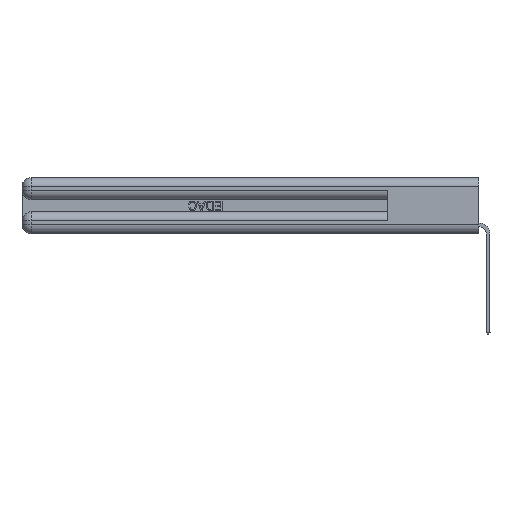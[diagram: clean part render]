
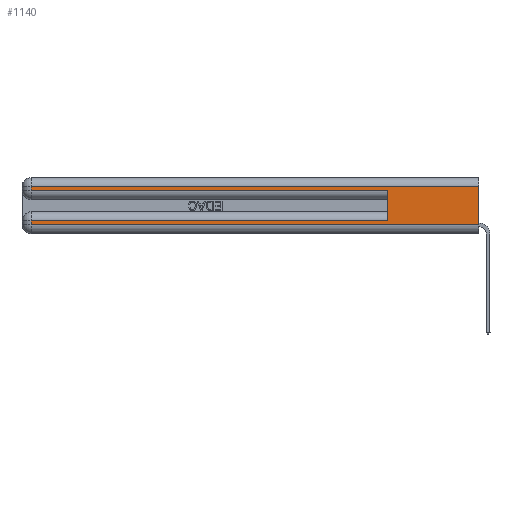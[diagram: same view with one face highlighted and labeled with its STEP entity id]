
A CAD part, left-side view. The second image highlights one B-rep face of the part: STEP entity #1140.
In plain terms, the highlighted planar face has unit normal (-1, 0, 0).
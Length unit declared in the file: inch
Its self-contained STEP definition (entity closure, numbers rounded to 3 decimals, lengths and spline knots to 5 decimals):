
#149 = VERTEX_POINT ( 'NONE', #10172 ) ;
#1140 = ADVANCED_FACE ( 'NONE', ( #12728 ), #4975, .F. ) ;
#1617 = VERTEX_POINT ( 'NONE', #30118 ) ;
#2623 = CARTESIAN_POINT ( 'NONE',  ( 0., 0., 0.06 ) ) ;
#4457 = LINE ( 'NONE', #31286, #9671 ) ;
#4912 = VERTEX_POINT ( 'NONE', #27541 ) ;
#4975 = PLANE ( 'NONE',  #32901 ) ;
#6109 = VECTOR ( 'NONE', #21089, 39.37008 ) ;
#6160 = ORIENTED_EDGE ( 'NONE', *, *, #14109, .T. ) ;
#6341 = ORIENTED_EDGE ( 'NONE', *, *, #18902, .T. ) ;
#6410 = VERTEX_POINT ( 'NONE', #9986 ) ;
#7077 = EDGE_CURVE ( 'NONE', #149, #32841, #21842, .T. ) ;
#7420 = DIRECTION ( 'NONE',  ( 0., -1., 0. ) ) ;
#8666 = VERTEX_POINT ( 'NONE', #9913 ) ;
#9593 = VECTOR ( 'NONE', #17671, 39.37008 ) ;
#9671 = VECTOR ( 'NONE', #20582, 39.37008 ) ;
#9913 = CARTESIAN_POINT ( 'NONE',  ( 0., 2.94, 0.06 ) ) ;
#9986 = CARTESIAN_POINT ( 'NONE',  ( 0., 2.94, 0.285 ) ) ;
#10080 = VECTOR ( 'NONE', #26228, 39.37008 ) ;
#10094 = DIRECTION ( 'NONE',  ( 0., 0., -1. ) ) ;
#10172 = CARTESIAN_POINT ( 'NONE',  ( 0., 0., 0.31 ) ) ;
#10383 = ORIENTED_EDGE ( 'NONE', *, *, #15410, .F. ) ;
#10410 = CARTESIAN_POINT ( 'NONE',  ( 0., 0., 0.37 ) ) ;
#10674 = VECTOR ( 'NONE', #7420, 39.37008 ) ;
#10763 = ORIENTED_EDGE ( 'NONE', *, *, #30979, .T. ) ;
#11105 = CARTESIAN_POINT ( 'NONE',  ( 0., 2.94, 0.37 ) ) ;
#12728 = FACE_OUTER_BOUND ( 'NONE', #19848, .T. ) ;
#13769 = CARTESIAN_POINT ( 'NONE',  ( 0., 2.94, 0.31 ) ) ;
#14002 = DIRECTION ( 'NONE',  ( 0., -1., 0. ) ) ;
#14109 = EDGE_CURVE ( 'NONE', #4912, #8666, #27395, .T. ) ;
#14332 = VERTEX_POINT ( 'NONE', #25302 ) ;
#14544 = EDGE_CURVE ( 'NONE', #6410, #14332, #28425, .T. ) ;
#14593 = ORIENTED_EDGE ( 'NONE', *, *, #30171, .T. ) ;
#15109 = CARTESIAN_POINT ( 'NONE',  ( 0., 0., 0.285 ) ) ;
#15410 = EDGE_CURVE ( 'NONE', #149, #25708, #21267, .T. ) ;
#15696 = DIRECTION ( 'NONE',  ( 1., 0., 0. ) ) ;
#17338 = VECTOR ( 'NONE', #24076, 39.37008 ) ;
#17671 = DIRECTION ( 'NONE',  ( 0., 0., -1. ) ) ;
#18320 = LINE ( 'NONE', #28848, #10080 ) ;
#18902 = EDGE_CURVE ( 'NONE', #1617, #4912, #4457, .T. ) ;
#19848 = EDGE_LOOP ( 'NONE', ( #10383, #24014, #10763, #33654, #32782, #6341, #6160, #14593 ) ) ;
#20227 = LINE ( 'NONE', #33742, #10674 ) ;
#20582 = DIRECTION ( 'NONE',  ( 0., 1., 0. ) ) ;
#21089 = DIRECTION ( 'NONE',  ( 0., 0., -1. ) ) ;
#21267 = LINE ( 'NONE', #10410, #6109 ) ;
#21655 = CARTESIAN_POINT ( 'NONE',  ( 0., 0., 0.31 ) ) ;
#21842 = LINE ( 'NONE', #21655, #33271 ) ;
#22771 = LINE ( 'NONE', #33657, #9593 ) ;
#24014 = ORIENTED_EDGE ( 'NONE', *, *, #7077, .T. ) ;
#24076 = DIRECTION ( 'NONE',  ( 0., 0., -1. ) ) ;
#25302 = CARTESIAN_POINT ( 'NONE',  ( 0., 0.6, 0.285 ) ) ;
#25708 = VERTEX_POINT ( 'NONE', #2623 ) ;
#26228 = DIRECTION ( 'NONE',  ( 0., 0., 1. ) ) ;
#27395 = LINE ( 'NONE', #11105, #17338 ) ;
#27541 = CARTESIAN_POINT ( 'NONE',  ( 0., 2.94, 0.085 ) ) ;
#28155 = EDGE_CURVE ( 'NONE', #1617, #14332, #18320, .T. ) ;
#28425 = LINE ( 'NONE', #15109, #28469 ) ;
#28469 = VECTOR ( 'NONE', #14002, 39.37008 ) ;
#28848 = CARTESIAN_POINT ( 'NONE',  ( 0., 0.6, 0.145 ) ) ;
#29217 = DIRECTION ( 'NONE',  ( 0., 1., 0. ) ) ;
#30118 = CARTESIAN_POINT ( 'NONE',  ( 0., 0.6, 0.085 ) ) ;
#30171 = EDGE_CURVE ( 'NONE', #8666, #25708, #20227, .T. ) ;
#30979 = EDGE_CURVE ( 'NONE', #32841, #6410, #22771, .T. ) ;
#31286 = CARTESIAN_POINT ( 'NONE',  ( 0., 0., 0.085 ) ) ;
#32782 = ORIENTED_EDGE ( 'NONE', *, *, #28155, .F. ) ;
#32841 = VERTEX_POINT ( 'NONE', #13769 ) ;
#32901 = AXIS2_PLACEMENT_3D ( 'NONE', #34117, #15696, #10094 ) ;
#33271 = VECTOR ( 'NONE', #29217, 39.37008 ) ;
#33654 = ORIENTED_EDGE ( 'NONE', *, *, #14544, .T. ) ;
#33657 = CARTESIAN_POINT ( 'NONE',  ( 0., 2.94, 0.37 ) ) ;
#33742 = CARTESIAN_POINT ( 'NONE',  ( 0., 0., 0.06 ) ) ;
#34117 = CARTESIAN_POINT ( 'NONE',  ( 0., 0., 0.37 ) ) ;
